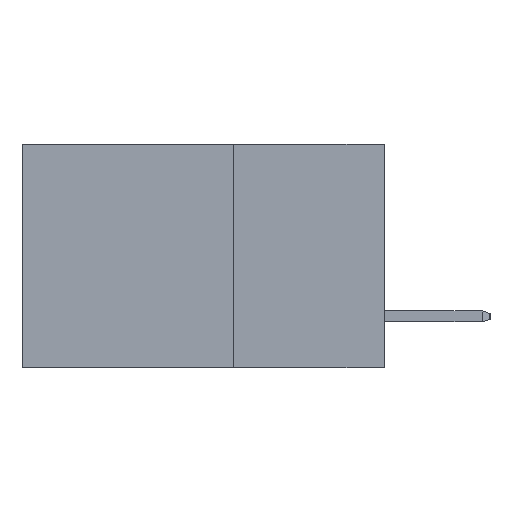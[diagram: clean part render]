
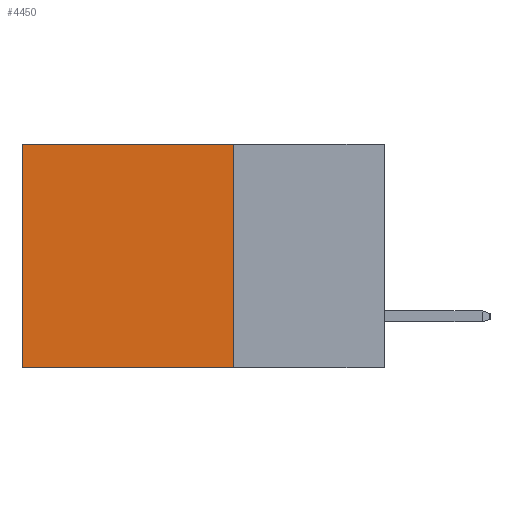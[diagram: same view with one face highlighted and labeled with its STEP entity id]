
A CAD part, left-side view. The second image highlights one B-rep face of the part: STEP entity #4450.
In plain terms, the highlighted planar face has unit normal (-1, 0, 0).
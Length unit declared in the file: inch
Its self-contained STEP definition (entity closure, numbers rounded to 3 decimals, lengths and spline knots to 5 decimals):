
#601 = EDGE_CURVE ( 'NONE', #6645, #4587, #7372, .T. ) ;
#814 = LINE ( 'NONE', #9809, #10436 ) ;
#2340 = CARTESIAN_POINT ( 'NONE',  ( 0.298, 0.6, 0. ) ) ;
#2815 = VERTEX_POINT ( 'NONE', #2340 ) ;
#4071 = EDGE_CURVE ( 'NONE', #2815, #4587, #9563, .T. ) ;
#4249 = EDGE_LOOP ( 'NONE', ( #19528, #16678, #21099, #6944 ) ) ;
#4450 = ADVANCED_FACE ( 'NONE', ( #5675 ), #8595, .F. ) ;
#4565 = CARTESIAN_POINT ( 'NONE',  ( 0.298, 0.6, -0.37 ) ) ;
#4587 = VERTEX_POINT ( 'NONE', #4565 ) ;
#4894 = AXIS2_PLACEMENT_3D ( 'NONE', #8745, #8560, #8534 ) ;
#5675 = FACE_OUTER_BOUND ( 'NONE', #4249, .T. ) ;
#6645 = VERTEX_POINT ( 'NONE', #10602 ) ;
#6944 = ORIENTED_EDGE ( 'NONE', *, *, #18292, .T. ) ;
#7372 = LINE ( 'NONE', #15616, #21810 ) ;
#8534 = DIRECTION ( 'NONE',  ( 0., 0., -1. ) ) ;
#8560 = DIRECTION ( 'NONE',  ( 1., 0., 0. ) ) ;
#8595 = PLANE ( 'NONE',  #4894 ) ;
#8745 = CARTESIAN_POINT ( 'NONE',  ( 0.298, 0.25, 0. ) ) ;
#9563 = LINE ( 'NONE', #20850, #14658 ) ;
#9809 = CARTESIAN_POINT ( 'NONE',  ( 0.298, 0.25, 0. ) ) ;
#10436 = VECTOR ( 'NONE', #17380, 39.37008 ) ;
#10570 = VECTOR ( 'NONE', #20115, 39.37008 ) ;
#10602 = CARTESIAN_POINT ( 'NONE',  ( 0.298, 0.25, -0.37 ) ) ;
#14523 = CARTESIAN_POINT ( 'NONE',  ( 0.298, 0.25, 0. ) ) ;
#14658 = VECTOR ( 'NONE', #20874, 39.37008 ) ;
#15616 = CARTESIAN_POINT ( 'NONE',  ( 0.298, 0.25, -0.37 ) ) ;
#16418 = VERTEX_POINT ( 'NONE', #23736 ) ;
#16678 = ORIENTED_EDGE ( 'NONE', *, *, #601, .F. ) ;
#17380 = DIRECTION ( 'NONE',  ( 0., 0., -1. ) ) ;
#18292 = EDGE_CURVE ( 'NONE', #16418, #2815, #24294, .T. ) ;
#19528 = ORIENTED_EDGE ( 'NONE', *, *, #4071, .T. ) ;
#20115 = DIRECTION ( 'NONE',  ( 0., 1., 0. ) ) ;
#20850 = CARTESIAN_POINT ( 'NONE',  ( 0.298, 0.6, 0. ) ) ;
#20874 = DIRECTION ( 'NONE',  ( 0., 0., -1. ) ) ;
#21035 = EDGE_CURVE ( 'NONE', #16418, #6645, #814, .T. ) ;
#21099 = ORIENTED_EDGE ( 'NONE', *, *, #21035, .F. ) ;
#21292 = DIRECTION ( 'NONE',  ( 0., 1., 0. ) ) ;
#21810 = VECTOR ( 'NONE', #21292, 39.37008 ) ;
#23736 = CARTESIAN_POINT ( 'NONE',  ( 0.298, 0.25, 0. ) ) ;
#24294 = LINE ( 'NONE', #14523, #10570 ) ;
